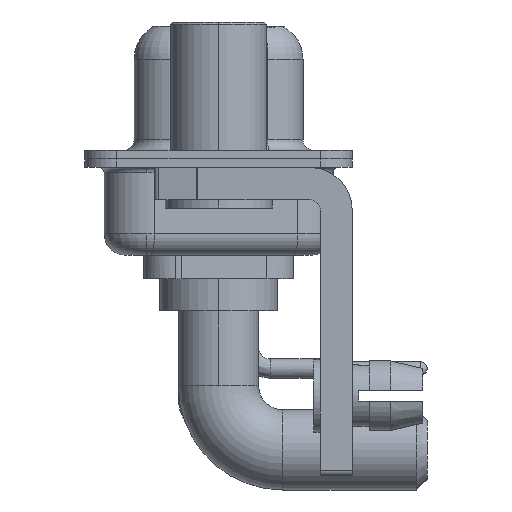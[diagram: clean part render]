
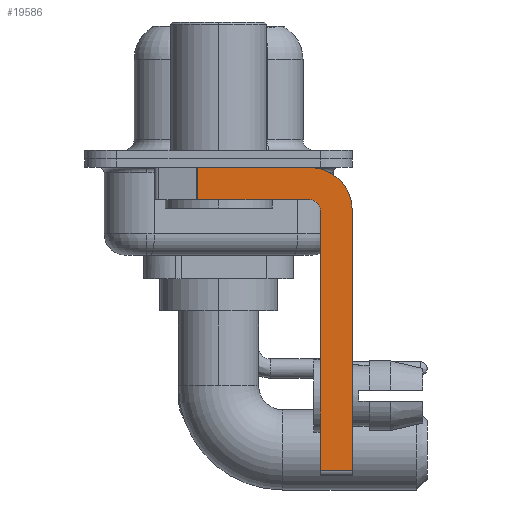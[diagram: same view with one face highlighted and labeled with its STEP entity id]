
A CAD part, left-side view. The second image highlights one B-rep face of the part: STEP entity #19586.
In plain terms, the highlighted planar face has unit normal (-1, 0, 0).
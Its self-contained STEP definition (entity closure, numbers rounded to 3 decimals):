
#85 = ORIENTED_EDGE ( 'NONE', *, *, #4078, .F. ) ;
#139 = EDGE_CURVE ( 'NONE', #2437, #13834, #14574, .T. ) ;
#281 = EDGE_CURVE ( 'NONE', #10491, #2943, #6070, .T. ) ;
#871 = ORIENTED_EDGE ( 'NONE', *, *, #8324, .F. ) ;
#1141 = AXIS2_PLACEMENT_3D ( 'NONE', #14282, #15868, #21352 ) ;
#1342 = CARTESIAN_POINT ( 'NONE',  ( -2.9, 0.978, -0.4 ) ) ;
#2437 = VERTEX_POINT ( 'NONE', #8993 ) ;
#2503 = DIRECTION ( 'NONE',  ( 0., 0., -1. ) ) ;
#2756 = CARTESIAN_POINT ( 'NONE',  ( -2.9, -6.25, -2.4 ) ) ;
#2943 = VERTEX_POINT ( 'NONE', #10713 ) ;
#3477 = CARTESIAN_POINT ( 'NONE',  ( -2.9, -4.25, -0.4 ) ) ;
#4019 = VERTEX_POINT ( 'NONE', #6130 ) ;
#4078 = EDGE_CURVE ( 'NONE', #14839, #10491, #10162, .T. ) ;
#4139 = ORIENTED_EDGE ( 'NONE', *, *, #18397, .F. ) ;
#4359 = CIRCLE ( 'NONE', #18133, 0.5 ) ;
#4570 = DIRECTION ( 'NONE',  ( 1., 0., 0. ) ) ;
#6070 = LINE ( 'NONE', #13598, #7528 ) ;
#6130 = CARTESIAN_POINT ( 'NONE',  ( -2.9, -4.75, -2.4 ) ) ;
#6749 = CARTESIAN_POINT ( 'NONE',  ( -2.9, 3., -0.4 ) ) ;
#7528 = VECTOR ( 'NONE', #7932, 1000. ) ;
#7571 = VECTOR ( 'NONE', #22524, 1000. ) ;
#7932 = DIRECTION ( 'NONE',  ( 0., 0., -1. ) ) ;
#8136 = ORIENTED_EDGE ( 'NONE', *, *, #139, .F. ) ;
#8324 = EDGE_CURVE ( 'NONE', #17140, #4019, #14585, .T. ) ;
#8359 = VERTEX_POINT ( 'NONE', #1342 ) ;
#8602 = EDGE_CURVE ( 'NONE', #8359, #13834, #9423, .T. ) ;
#8993 = CARTESIAN_POINT ( 'NONE',  ( -2.9, -4.25, -1.9 ) ) ;
#9423 = LINE ( 'NONE', #13980, #21807 ) ;
#9627 = DIRECTION ( 'NONE',  ( -1., 0., 0. ) ) ;
#9919 = AXIS2_PLACEMENT_3D ( 'NONE', #19383, #4570, #2503 ) ;
#10162 = CIRCLE ( 'NONE', #1141, 2. ) ;
#10491 = VERTEX_POINT ( 'NONE', #2756 ) ;
#10713 = CARTESIAN_POINT ( 'NONE',  ( -2.9, -6.25, -14.55 ) ) ;
#11160 = CARTESIAN_POINT ( 'NONE',  ( -2.9, -4.25, -1.9 ) ) ;
#11462 = VECTOR ( 'NONE', #14298, 1000. ) ;
#11614 = DIRECTION ( 'NONE',  ( 0., 0., 1. ) ) ;
#11855 = CARTESIAN_POINT ( 'NONE',  ( -2.9, -4.25, -14.55 ) ) ;
#11944 = VECTOR ( 'NONE', #24017, 1000. ) ;
#12322 = EDGE_LOOP ( 'NONE', ( #4139, #15934, #8136, #16153, #871, #12938, #24363, #85 ) ) ;
#12791 = CARTESIAN_POINT ( 'NONE',  ( -2.9, 0.978, -1.9 ) ) ;
#12938 = ORIENTED_EDGE ( 'NONE', *, *, #15059, .T. ) ;
#13598 = CARTESIAN_POINT ( 'NONE',  ( -2.9, -6.25, -2.4 ) ) ;
#13834 = VERTEX_POINT ( 'NONE', #12791 ) ;
#13980 = CARTESIAN_POINT ( 'NONE',  ( -2.9, 0.978, -1.9 ) ) ;
#14282 = CARTESIAN_POINT ( 'NONE',  ( -2.9, -4.25, -2.4 ) ) ;
#14298 = DIRECTION ( 'NONE',  ( 0., -1., 0. ) ) ;
#14404 = LINE ( 'NONE', #6749, #11462 ) ;
#14574 = LINE ( 'NONE', #11160, #7571 ) ;
#14585 = LINE ( 'NONE', #22172, #11944 ) ;
#14839 = VERTEX_POINT ( 'NONE', #3477 ) ;
#15059 = EDGE_CURVE ( 'NONE', #17140, #2943, #23228, .T. ) ;
#15868 = DIRECTION ( 'NONE',  ( 1., 0., 0. ) ) ;
#15934 = ORIENTED_EDGE ( 'NONE', *, *, #8602, .T. ) ;
#16153 = ORIENTED_EDGE ( 'NONE', *, *, #21407, .F. ) ;
#17140 = VERTEX_POINT ( 'NONE', #20626 ) ;
#17377 = PLANE ( 'NONE',  #9919 ) ;
#17428 = DIRECTION ( 'NONE',  ( 0., 0., -1. ) ) ;
#17621 = DIRECTION ( 'NONE',  ( 0., -1., 0. ) ) ;
#18133 = AXIS2_PLACEMENT_3D ( 'NONE', #19005, #9627, #11614 ) ;
#18397 = EDGE_CURVE ( 'NONE', #8359, #14839, #14404, .T. ) ;
#19005 = CARTESIAN_POINT ( 'NONE',  ( -2.9, -4.25, -2.4 ) ) ;
#19383 = CARTESIAN_POINT ( 'NONE',  ( -2.9, -4.25, -2.4 ) ) ;
#19586 = ADVANCED_FACE ( 'NONE', ( #23347 ), #17377, .F. ) ;
#20626 = CARTESIAN_POINT ( 'NONE',  ( -2.9, -4.75, -14.55 ) ) ;
#21352 = DIRECTION ( 'NONE',  ( 0., 0., -1. ) ) ;
#21407 = EDGE_CURVE ( 'NONE', #4019, #2437, #4359, .T. ) ;
#21807 = VECTOR ( 'NONE', #17428, 1000. ) ;
#22172 = CARTESIAN_POINT ( 'NONE',  ( -2.9, -4.75, -14.8 ) ) ;
#22524 = DIRECTION ( 'NONE',  ( 0., 1., 0. ) ) ;
#23214 = VECTOR ( 'NONE', #17621, 1000. ) ;
#23228 = LINE ( 'NONE', #11855, #23214 ) ;
#23347 = FACE_OUTER_BOUND ( 'NONE', #12322, .T. ) ;
#24017 = DIRECTION ( 'NONE',  ( 0., 0., 1. ) ) ;
#24363 = ORIENTED_EDGE ( 'NONE', *, *, #281, .F. ) ;
